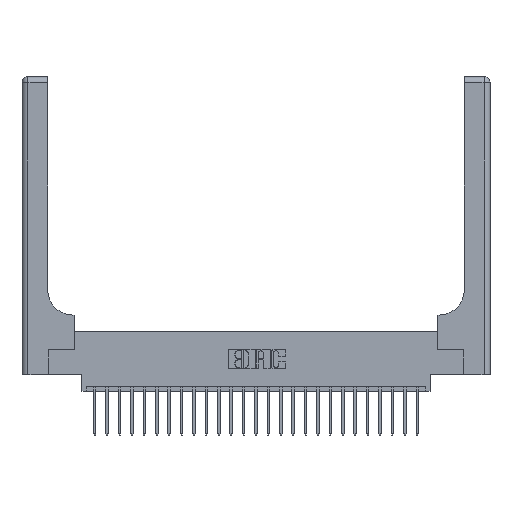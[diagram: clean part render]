
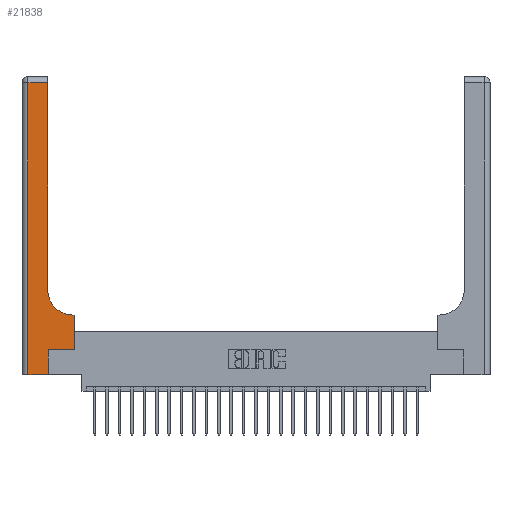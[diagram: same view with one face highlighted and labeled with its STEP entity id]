
A CAD part, top view. The second image highlights one B-rep face of the part: STEP entity #21838.
In plain terms, the highlighted planar face has unit normal (0, 0, 1).
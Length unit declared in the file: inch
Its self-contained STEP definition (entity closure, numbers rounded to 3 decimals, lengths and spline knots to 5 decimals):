
#139 = EDGE_CURVE ( 'NONE', #18315, #10824, #24666, .T. ) ;
#391 = DIRECTION ( 'NONE',  ( 0., 0., -1. ) ) ;
#475 = CARTESIAN_POINT ( 'NONE',  ( 0.06, 0., 0.37 ) ) ;
#746 = EDGE_CURVE ( 'NONE', #5840, #19093, #21512, .T. ) ;
#822 = AXIS2_PLACEMENT_3D ( 'NONE', #898, #12641, #5153 ) ;
#898 = CARTESIAN_POINT ( 'NONE',  ( 0., 3., 0.37 ) ) ;
#1013 = ORIENTED_EDGE ( 'NONE', *, *, #7167, .T. ) ;
#1093 = DIRECTION ( 'NONE',  ( 0., 1., 0. ) ) ;
#1219 = VECTOR ( 'NONE', #10547, 39.37008 ) ;
#1679 = VECTOR ( 'NONE', #15200, 39.37008 ) ;
#2623 = CARTESIAN_POINT ( 'NONE',  ( 0.265, 0., 0.37 ) ) ;
#2846 = ORIENTED_EDGE ( 'NONE', *, *, #4579, .T. ) ;
#3040 = CARTESIAN_POINT ( 'NONE',  ( 0., 0., 0.37 ) ) ;
#3362 = CARTESIAN_POINT ( 'NONE',  ( 0.26, 0.85, 0.37 ) ) ;
#3796 = VERTEX_POINT ( 'NONE', #3362 ) ;
#4116 = CIRCLE ( 'NONE', #7810, 0.25 ) ;
#4579 = EDGE_CURVE ( 'NONE', #15563, #12004, #17465, .T. ) ;
#5153 = DIRECTION ( 'NONE',  ( -1., 0., 0. ) ) ;
#5209 = LINE ( 'NONE', #12696, #16025 ) ;
#5840 = VERTEX_POINT ( 'NONE', #24379 ) ;
#6051 = EDGE_CURVE ( 'NONE', #3796, #15563, #5209, .T. ) ;
#6826 = PLANE ( 'NONE',  #822 ) ;
#6918 = LINE ( 'NONE', #20410, #1219 ) ;
#7060 = CARTESIAN_POINT ( 'NONE',  ( 0.265, 0.25, 0.37 ) ) ;
#7167 = EDGE_CURVE ( 'NONE', #12004, #18315, #8183, .T. ) ;
#7684 = VECTOR ( 'NONE', #21038, 39.37008 ) ;
#7810 = AXIS2_PLACEMENT_3D ( 'NONE', #14187, #391, #12117 ) ;
#7895 = DIRECTION ( 'NONE',  ( -1., 0., 0. ) ) ;
#8015 = VERTEX_POINT ( 'NONE', #23627 ) ;
#8183 = LINE ( 'NONE', #22186, #8352 ) ;
#8352 = VECTOR ( 'NONE', #21932, 39.37008 ) ;
#8804 = VECTOR ( 'NONE', #21168, 39.37008 ) ;
#9490 = CARTESIAN_POINT ( 'NONE',  ( 0., 2.94, 0.37 ) ) ;
#10547 = DIRECTION ( 'NONE',  ( 0., 1., 0. ) ) ;
#10824 = VERTEX_POINT ( 'NONE', #2623 ) ;
#10931 = DIRECTION ( 'NONE',  ( 1., 0., 0. ) ) ;
#11228 = FACE_OUTER_BOUND ( 'NONE', #17763, .T. ) ;
#11297 = VERTEX_POINT ( 'NONE', #7060 ) ;
#12004 = VERTEX_POINT ( 'NONE', #20588 ) ;
#12117 = DIRECTION ( 'NONE',  ( 1., 0., 0. ) ) ;
#12349 = ORIENTED_EDGE ( 'NONE', *, *, #13246, .T. ) ;
#12641 = DIRECTION ( 'NONE',  ( 0., 0., -1. ) ) ;
#12696 = CARTESIAN_POINT ( 'NONE',  ( 0.26, 3., 0.37 ) ) ;
#13149 = CARTESIAN_POINT ( 'NONE',  ( 0.265, 0.25, 0.37 ) ) ;
#13246 = EDGE_CURVE ( 'NONE', #10824, #11297, #18865, .T. ) ;
#13803 = ORIENTED_EDGE ( 'NONE', *, *, #21678, .T. ) ;
#13948 = ORIENTED_EDGE ( 'NONE', *, *, #20989, .T. ) ;
#13960 = CARTESIAN_POINT ( 'NONE',  ( 0.26, 0.6, 0.37 ) ) ;
#14187 = CARTESIAN_POINT ( 'NONE',  ( 0.51, 0.85, 0.37 ) ) ;
#14386 = ORIENTED_EDGE ( 'NONE', *, *, #139, .T. ) ;
#15107 = VECTOR ( 'NONE', #10931, 39.37008 ) ;
#15200 = DIRECTION ( 'NONE',  ( 1., 0., 0. ) ) ;
#15563 = VERTEX_POINT ( 'NONE', #15590 ) ;
#15590 = CARTESIAN_POINT ( 'NONE',  ( 0.26, 2.94, 0.37 ) ) ;
#15625 = ORIENTED_EDGE ( 'NONE', *, *, #6051, .T. ) ;
#15701 = LINE ( 'NONE', #13149, #1679 ) ;
#16025 = VECTOR ( 'NONE', #1093, 39.37008 ) ;
#16929 = CARTESIAN_POINT ( 'NONE',  ( 0.51, 0.6, 0.37 ) ) ;
#17465 = LINE ( 'NONE', #9490, #8804 ) ;
#17763 = EDGE_LOOP ( 'NONE', ( #15625, #2846, #1013, #14386, #12349, #18233, #13948, #19153, #13803 ) ) ;
#18233 = ORIENTED_EDGE ( 'NONE', *, *, #20775, .T. ) ;
#18315 = VERTEX_POINT ( 'NONE', #475 ) ;
#18865 = LINE ( 'NONE', #18997, #7684 ) ;
#18997 = CARTESIAN_POINT ( 'NONE',  ( 0.265, 0., 0.37 ) ) ;
#19093 = VERTEX_POINT ( 'NONE', #16929 ) ;
#19153 = ORIENTED_EDGE ( 'NONE', *, *, #746, .T. ) ;
#20410 = CARTESIAN_POINT ( 'NONE',  ( 0.528, 0.25, 0.37 ) ) ;
#20588 = CARTESIAN_POINT ( 'NONE',  ( 0.06, 2.94, 0.37 ) ) ;
#20775 = EDGE_CURVE ( 'NONE', #11297, #8015, #15701, .T. ) ;
#20989 = EDGE_CURVE ( 'NONE', #8015, #5840, #6918, .T. ) ;
#21038 = DIRECTION ( 'NONE',  ( 0., 1., 0. ) ) ;
#21168 = DIRECTION ( 'NONE',  ( -1., 0., 0. ) ) ;
#21512 = LINE ( 'NONE', #13960, #24998 ) ;
#21678 = EDGE_CURVE ( 'NONE', #19093, #3796, #4116, .T. ) ;
#21838 = ADVANCED_FACE ( 'NONE', ( #11228 ), #6826, .F. ) ;
#21932 = DIRECTION ( 'NONE',  ( 0., -1., 0. ) ) ;
#22186 = CARTESIAN_POINT ( 'NONE',  ( 0.06, 3., 0.37 ) ) ;
#23627 = CARTESIAN_POINT ( 'NONE',  ( 0.528, 0.25, 0.37 ) ) ;
#24379 = CARTESIAN_POINT ( 'NONE',  ( 0.528, 0.6, 0.37 ) ) ;
#24666 = LINE ( 'NONE', #3040, #15107 ) ;
#24998 = VECTOR ( 'NONE', #7895, 39.37008 ) ;
